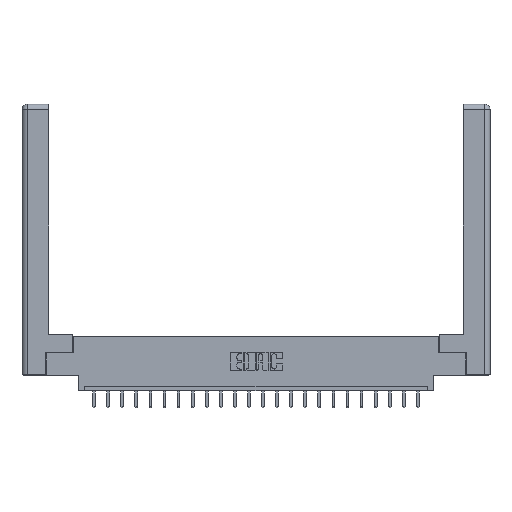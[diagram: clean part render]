
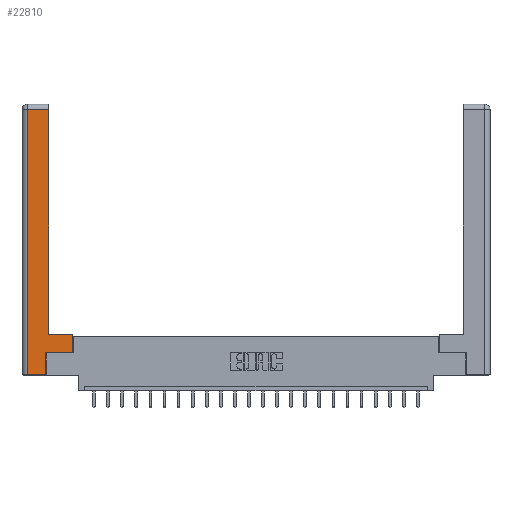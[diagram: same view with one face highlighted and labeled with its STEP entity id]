
A CAD part, top view. The second image highlights one B-rep face of the part: STEP entity #22810.
In plain terms, the highlighted planar face has unit normal (0, 0, 1).
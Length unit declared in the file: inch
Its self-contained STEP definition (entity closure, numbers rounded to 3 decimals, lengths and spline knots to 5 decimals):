
#28 = DIRECTION ( 'NONE',  ( -1., 0., 0. ) ) ;
#317 = LINE ( 'NONE', #16862, #18697 ) ;
#464 = ORIENTED_EDGE ( 'NONE', *, *, #9589, .T. ) ;
#591 = LINE ( 'NONE', #2950, #10850 ) ;
#825 = CARTESIAN_POINT ( 'NONE',  ( 0.565, 0.245, 0. ) ) ;
#988 = CARTESIAN_POINT ( 'NONE',  ( 0.265, 0.245, 0. ) ) ;
#1158 = DIRECTION ( 'NONE',  ( 0., 1., 0. ) ) ;
#1714 = VERTEX_POINT ( 'NONE', #10752 ) ;
#2950 = CARTESIAN_POINT ( 'NONE',  ( 0.265, 0., 0. ) ) ;
#3107 = VECTOR ( 'NONE', #1158, 39.37008 ) ;
#3490 = ORIENTED_EDGE ( 'NONE', *, *, #20245, .T. ) ;
#3578 = LINE ( 'NONE', #988, #17195 ) ;
#3898 = LINE ( 'NONE', #19105, #12779 ) ;
#3899 = VERTEX_POINT ( 'NONE', #17939 ) ;
#4309 = DIRECTION ( 'NONE',  ( 0., -1., 0. ) ) ;
#4374 = DIRECTION ( 'NONE',  ( 0., 0., -1. ) ) ;
#6180 = LINE ( 'NONE', #18911, #3107 ) ;
#6415 = EDGE_CURVE ( 'NONE', #16301, #21200, #317, .T. ) ;
#6615 = DIRECTION ( 'NONE',  ( -1., 0., 0. ) ) ;
#6869 = DIRECTION ( 'NONE',  ( 0., 1., 0. ) ) ;
#7268 = VERTEX_POINT ( 'NONE', #825 ) ;
#7549 = CARTESIAN_POINT ( 'NONE',  ( 0.0615, 0., 0. ) ) ;
#7853 = VERTEX_POINT ( 'NONE', #12646 ) ;
#8298 = DIRECTION ( 'NONE',  ( 1., 0., 0. ) ) ;
#8380 = EDGE_CURVE ( 'NONE', #13982, #1714, #13711, .T. ) ;
#8649 = EDGE_LOOP ( 'NONE', ( #464, #20430, #9799, #3490, #19590, #16705, #13934, #15791 ) ) ;
#9589 = EDGE_CURVE ( 'NONE', #1714, #22579, #6180, .T. ) ;
#9799 = ORIENTED_EDGE ( 'NONE', *, *, #6415, .T. ) ;
#9950 = EDGE_CURVE ( 'NONE', #7853, #7268, #11718, .T. ) ;
#10271 = CARTESIAN_POINT ( 'NONE',  ( 0.295, 2.94, 0. ) ) ;
#10752 = CARTESIAN_POINT ( 'NONE',  ( 0.295, 0.45, 0. ) ) ;
#10850 = VECTOR ( 'NONE', #8298, 39.37008 ) ;
#11199 = EDGE_CURVE ( 'NONE', #3899, #7853, #3578, .T. ) ;
#11404 = EDGE_CURVE ( 'NONE', #22579, #16301, #20176, .T. ) ;
#11718 = LINE ( 'NONE', #15431, #22340 ) ;
#12646 = CARTESIAN_POINT ( 'NONE',  ( 0.265, 0.245, 0. ) ) ;
#12752 = AXIS2_PLACEMENT_3D ( 'NONE', #13228, #4374, #15010 ) ;
#12779 = VECTOR ( 'NONE', #6869, 39.37008 ) ;
#13228 = CARTESIAN_POINT ( 'NONE',  ( 0., 0., 0. ) ) ;
#13560 = CARTESIAN_POINT ( 'NONE',  ( 0.0615, 2.94, 0. ) ) ;
#13711 = LINE ( 'NONE', #14400, #17057 ) ;
#13934 = ORIENTED_EDGE ( 'NONE', *, *, #20680, .T. ) ;
#13982 = VERTEX_POINT ( 'NONE', #18512 ) ;
#14122 = CARTESIAN_POINT ( 'NONE',  ( 0.0615, 2.94, 0. ) ) ;
#14400 = CARTESIAN_POINT ( 'NONE',  ( 0.295, 0.45, 0. ) ) ;
#15010 = DIRECTION ( 'NONE',  ( -1., 0., 0. ) ) ;
#15431 = CARTESIAN_POINT ( 'NONE',  ( 0.565, 0.245, 0. ) ) ;
#15791 = ORIENTED_EDGE ( 'NONE', *, *, #8380, .T. ) ;
#16301 = VERTEX_POINT ( 'NONE', #14122 ) ;
#16705 = ORIENTED_EDGE ( 'NONE', *, *, #9950, .T. ) ;
#16862 = CARTESIAN_POINT ( 'NONE',  ( 0.0615, 0., 0. ) ) ;
#16988 = DIRECTION ( 'NONE',  ( 0., 1., 0. ) ) ;
#17015 = FACE_OUTER_BOUND ( 'NONE', #8649, .T. ) ;
#17057 = VECTOR ( 'NONE', #28, 39.37008 ) ;
#17195 = VECTOR ( 'NONE', #16988, 39.37008 ) ;
#17939 = CARTESIAN_POINT ( 'NONE',  ( 0.265, 0., 0. ) ) ;
#18512 = CARTESIAN_POINT ( 'NONE',  ( 0.565, 0.45, 0. ) ) ;
#18697 = VECTOR ( 'NONE', #4309, 39.37008 ) ;
#18911 = CARTESIAN_POINT ( 'NONE',  ( 0.295, 3., 0. ) ) ;
#19105 = CARTESIAN_POINT ( 'NONE',  ( 0.565, 0.45, 0. ) ) ;
#19590 = ORIENTED_EDGE ( 'NONE', *, *, #11199, .T. ) ;
#20176 = LINE ( 'NONE', #13560, #22968 ) ;
#20245 = EDGE_CURVE ( 'NONE', #21200, #3899, #591, .T. ) ;
#20316 = PLANE ( 'NONE',  #12752 ) ;
#20430 = ORIENTED_EDGE ( 'NONE', *, *, #11404, .T. ) ;
#20680 = EDGE_CURVE ( 'NONE', #7268, #13982, #3898, .T. ) ;
#20799 = DIRECTION ( 'NONE',  ( 1., 0., 0. ) ) ;
#21200 = VERTEX_POINT ( 'NONE', #7549 ) ;
#22340 = VECTOR ( 'NONE', #20799, 39.37008 ) ;
#22579 = VERTEX_POINT ( 'NONE', #10271 ) ;
#22810 = ADVANCED_FACE ( 'NONE', ( #17015 ), #20316, .F. ) ;
#22968 = VECTOR ( 'NONE', #6615, 39.37008 ) ;
